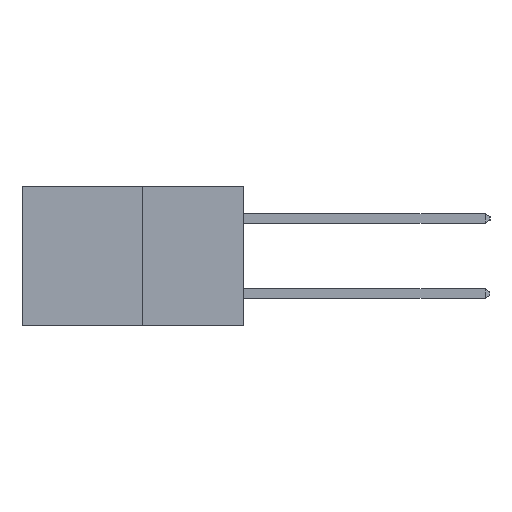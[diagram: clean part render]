
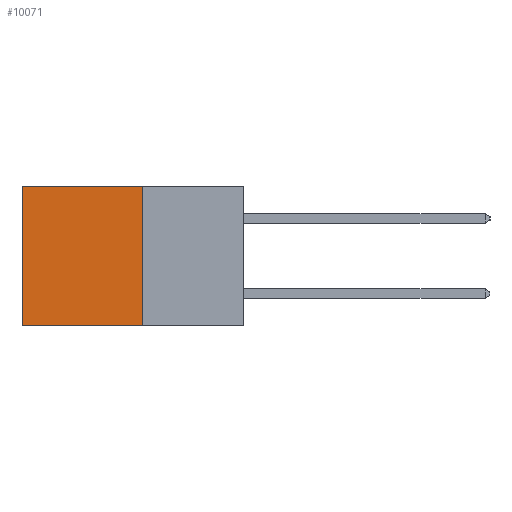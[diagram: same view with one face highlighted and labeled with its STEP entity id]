
A CAD part, left-side view. The second image highlights one B-rep face of the part: STEP entity #10071.
In plain terms, the highlighted planar face has unit normal (-1, 0, 0).
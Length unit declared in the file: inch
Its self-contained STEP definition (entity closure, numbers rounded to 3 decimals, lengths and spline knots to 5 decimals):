
#256 = EDGE_CURVE ( 'NONE', #6556, #12191, #2310, .T. ) ;
#1353 = ORIENTED_EDGE ( 'NONE', *, *, #256, .T. ) ;
#1537 = ORIENTED_EDGE ( 'NONE', *, *, #14279, .F. ) ;
#1955 = ORIENTED_EDGE ( 'NONE', *, *, #6387, .F. ) ;
#2310 = LINE ( 'NONE', #12384, #14693 ) ;
#2514 = VECTOR ( 'NONE', #12394, 39.37008 ) ;
#3066 = CARTESIAN_POINT ( 'NONE',  ( 0.277, 0.27, -0.37 ) ) ;
#4603 = EDGE_CURVE ( 'NONE', #4877, #6556, #15059, .T. ) ;
#4877 = VERTEX_POINT ( 'NONE', #12060 ) ;
#5255 = ORIENTED_EDGE ( 'NONE', *, *, #4603, .T. ) ;
#5551 = DIRECTION ( 'NONE',  ( 1., 0., 0. ) ) ;
#5732 = LINE ( 'NONE', #3066, #2514 ) ;
#5814 = DIRECTION ( 'NONE',  ( 0., 1., 0. ) ) ;
#6140 = CARTESIAN_POINT ( 'NONE',  ( 0.277, 0.27, 0. ) ) ;
#6387 = EDGE_CURVE ( 'NONE', #4877, #12152, #13487, .T. ) ;
#6556 = VERTEX_POINT ( 'NONE', #7429 ) ;
#7429 = CARTESIAN_POINT ( 'NONE',  ( 0.277, 0.59, 0. ) ) ;
#7620 = CARTESIAN_POINT ( 'NONE',  ( 0.277, 0.27, -0.37 ) ) ;
#7723 = VECTOR ( 'NONE', #8642, 39.37008 ) ;
#7842 = PLANE ( 'NONE',  #14409 ) ;
#8642 = DIRECTION ( 'NONE',  ( 0., 0., -1. ) ) ;
#8646 = CARTESIAN_POINT ( 'NONE',  ( 0.277, 0.27, -0.37 ) ) ;
#10071 = ADVANCED_FACE ( 'NONE', ( #11034 ), #7842, .F. ) ;
#10146 = DIRECTION ( 'NONE',  ( 0., 0., -1. ) ) ;
#11034 = FACE_OUTER_BOUND ( 'NONE', #11719, .T. ) ;
#11719 = EDGE_LOOP ( 'NONE', ( #1353, #1537, #1955, #5255 ) ) ;
#12060 = CARTESIAN_POINT ( 'NONE',  ( 0.277, 0.27, 0. ) ) ;
#12107 = VECTOR ( 'NONE', #5814, 39.37008 ) ;
#12152 = VERTEX_POINT ( 'NONE', #7620 ) ;
#12191 = VERTEX_POINT ( 'NONE', #14509 ) ;
#12384 = CARTESIAN_POINT ( 'NONE',  ( 0.277, 0.59, -0.37 ) ) ;
#12394 = DIRECTION ( 'NONE',  ( 0., 1., 0. ) ) ;
#12473 = CARTESIAN_POINT ( 'NONE',  ( 0.277, 0.27, -0.37 ) ) ;
#13487 = LINE ( 'NONE', #8646, #7723 ) ;
#13815 = DIRECTION ( 'NONE',  ( 0., 0., -1. ) ) ;
#14279 = EDGE_CURVE ( 'NONE', #12152, #12191, #5732, .T. ) ;
#14409 = AXIS2_PLACEMENT_3D ( 'NONE', #12473, #5551, #13815 ) ;
#14509 = CARTESIAN_POINT ( 'NONE',  ( 0.277, 0.59, -0.37 ) ) ;
#14693 = VECTOR ( 'NONE', #10146, 39.37008 ) ;
#15059 = LINE ( 'NONE', #6140, #12107 ) ;
